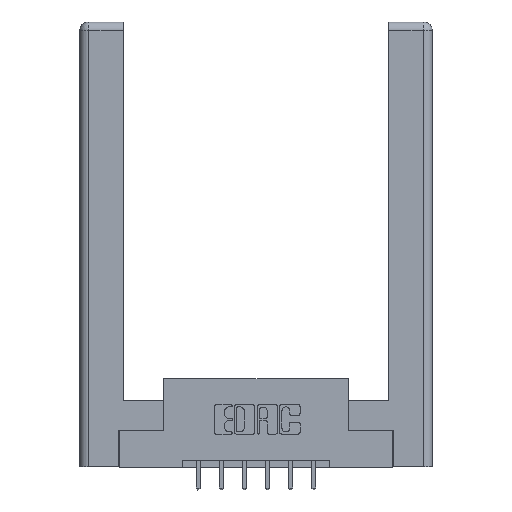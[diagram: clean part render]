
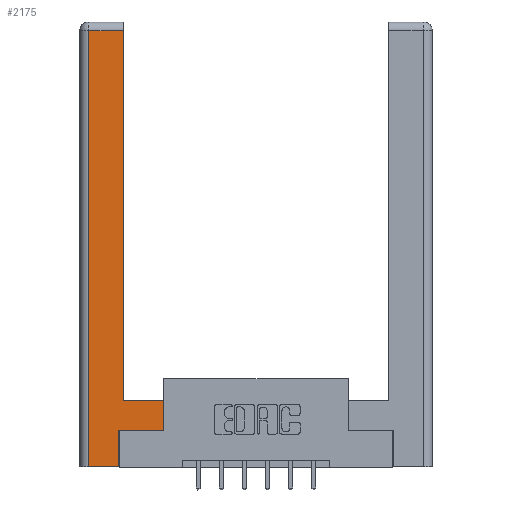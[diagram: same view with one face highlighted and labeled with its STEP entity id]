
A CAD part, top view. The second image highlights one B-rep face of the part: STEP entity #2175.
In plain terms, the highlighted planar face has unit normal (0, 0, 1).
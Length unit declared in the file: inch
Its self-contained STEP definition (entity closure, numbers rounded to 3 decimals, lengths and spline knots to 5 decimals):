
#752 = CARTESIAN_POINT ( 'NONE',  ( 0.565, 0.45, 0. ) ) ;
#913 = CARTESIAN_POINT ( 'NONE',  ( 0.265, 0.245, 0. ) ) ;
#1747 = DIRECTION ( 'NONE',  ( -1., 0., 0. ) ) ;
#2052 = VECTOR ( 'NONE', #7331, 39.37008 ) ;
#2130 = CARTESIAN_POINT ( 'NONE',  ( 0.565, 0.245, 0. ) ) ;
#2161 = LINE ( 'NONE', #4354, #8061 ) ;
#2175 = ADVANCED_FACE ( 'NONE', ( #11188 ), #3145, .F. ) ;
#2427 = ORIENTED_EDGE ( 'NONE', *, *, #8949, .T. ) ;
#2434 = AXIS2_PLACEMENT_3D ( 'NONE', #11329, #10508, #8608 ) ;
#2455 = DIRECTION ( 'NONE',  ( 1., 0., 0. ) ) ;
#2585 = DIRECTION ( 'NONE',  ( 0., 1., 0. ) ) ;
#2778 = LINE ( 'NONE', #3561, #4362 ) ;
#2809 = ORIENTED_EDGE ( 'NONE', *, *, #11724, .T. ) ;
#3145 = PLANE ( 'NONE',  #2434 ) ;
#3174 = CARTESIAN_POINT ( 'NONE',  ( 0.565, 0.45, 0. ) ) ;
#3182 = LINE ( 'NONE', #752, #7045 ) ;
#3274 = CARTESIAN_POINT ( 'NONE',  ( 0.565, 0.245, 0. ) ) ;
#3282 = CARTESIAN_POINT ( 'NONE',  ( 0.295, 3., 0. ) ) ;
#3401 = VECTOR ( 'NONE', #10220, 39.37008 ) ;
#3561 = CARTESIAN_POINT ( 'NONE',  ( 0.295, 0.45, 0. ) ) ;
#3845 = VERTEX_POINT ( 'NONE', #11019 ) ;
#3993 = LINE ( 'NONE', #3274, #4844 ) ;
#4039 = ORIENTED_EDGE ( 'NONE', *, *, #11626, .T. ) ;
#4081 = VERTEX_POINT ( 'NONE', #4514 ) ;
#4200 = EDGE_CURVE ( 'NONE', #3845, #5052, #5389, .T. ) ;
#4306 = VERTEX_POINT ( 'NONE', #2130 ) ;
#4354 = CARTESIAN_POINT ( 'NONE',  ( 0.0615, 0., 0. ) ) ;
#4362 = VECTOR ( 'NONE', #1747, 39.37008 ) ;
#4366 = CARTESIAN_POINT ( 'NONE',  ( 0.265, 0.245, 0. ) ) ;
#4504 = LINE ( 'NONE', #8221, #2052 ) ;
#4514 = CARTESIAN_POINT ( 'NONE',  ( 0.295, 0.45, 0. ) ) ;
#4537 = CARTESIAN_POINT ( 'NONE',  ( 0.295, 2.94, 0. ) ) ;
#4629 = LINE ( 'NONE', #3282, #7196 ) ;
#4844 = VECTOR ( 'NONE', #2455, 39.37008 ) ;
#4981 = LINE ( 'NONE', #5794, #3401 ) ;
#5052 = VERTEX_POINT ( 'NONE', #4366 ) ;
#5066 = EDGE_LOOP ( 'NONE', ( #6351, #4039, #8648, #5842, #5668, #2427, #11562, #2809 ) ) ;
#5129 = CARTESIAN_POINT ( 'NONE',  ( 0.0615, 0., 0. ) ) ;
#5389 = LINE ( 'NONE', #913, #6807 ) ;
#5656 = EDGE_CURVE ( 'NONE', #4081, #7437, #4629, .T. ) ;
#5668 = ORIENTED_EDGE ( 'NONE', *, *, #4200, .T. ) ;
#5681 = VERTEX_POINT ( 'NONE', #5129 ) ;
#5794 = CARTESIAN_POINT ( 'NONE',  ( 0.265, 0., 0. ) ) ;
#5842 = ORIENTED_EDGE ( 'NONE', *, *, #9416, .T. ) ;
#5855 = EDGE_CURVE ( 'NONE', #11805, #5681, #2161, .T. ) ;
#6351 = ORIENTED_EDGE ( 'NONE', *, *, #5656, .T. ) ;
#6687 = EDGE_CURVE ( 'NONE', #4306, #11184, #3182, .T. ) ;
#6807 = VECTOR ( 'NONE', #9266, 39.37008 ) ;
#7045 = VECTOR ( 'NONE', #2585, 39.37008 ) ;
#7196 = VECTOR ( 'NONE', #7937, 39.37008 ) ;
#7331 = DIRECTION ( 'NONE',  ( -1., 0., 0. ) ) ;
#7437 = VERTEX_POINT ( 'NONE', #4537 ) ;
#7937 = DIRECTION ( 'NONE',  ( 0., 1., 0. ) ) ;
#8061 = VECTOR ( 'NONE', #10838, 39.37008 ) ;
#8221 = CARTESIAN_POINT ( 'NONE',  ( 0.0615, 2.94, 0. ) ) ;
#8608 = DIRECTION ( 'NONE',  ( -1., 0., 0. ) ) ;
#8648 = ORIENTED_EDGE ( 'NONE', *, *, #5855, .T. ) ;
#8949 = EDGE_CURVE ( 'NONE', #5052, #4306, #3993, .T. ) ;
#9266 = DIRECTION ( 'NONE',  ( 0., 1., 0. ) ) ;
#9416 = EDGE_CURVE ( 'NONE', #5681, #3845, #4981, .T. ) ;
#10220 = DIRECTION ( 'NONE',  ( 1., 0., 0. ) ) ;
#10236 = CARTESIAN_POINT ( 'NONE',  ( 0.0615, 2.94, 0. ) ) ;
#10508 = DIRECTION ( 'NONE',  ( 0., 0., -1. ) ) ;
#10838 = DIRECTION ( 'NONE',  ( 0., -1., 0. ) ) ;
#11019 = CARTESIAN_POINT ( 'NONE',  ( 0.265, 0., 0. ) ) ;
#11184 = VERTEX_POINT ( 'NONE', #3174 ) ;
#11188 = FACE_OUTER_BOUND ( 'NONE', #5066, .T. ) ;
#11329 = CARTESIAN_POINT ( 'NONE',  ( 0., 0., 0. ) ) ;
#11562 = ORIENTED_EDGE ( 'NONE', *, *, #6687, .T. ) ;
#11626 = EDGE_CURVE ( 'NONE', #7437, #11805, #4504, .T. ) ;
#11724 = EDGE_CURVE ( 'NONE', #11184, #4081, #2778, .T. ) ;
#11805 = VERTEX_POINT ( 'NONE', #10236 ) ;
